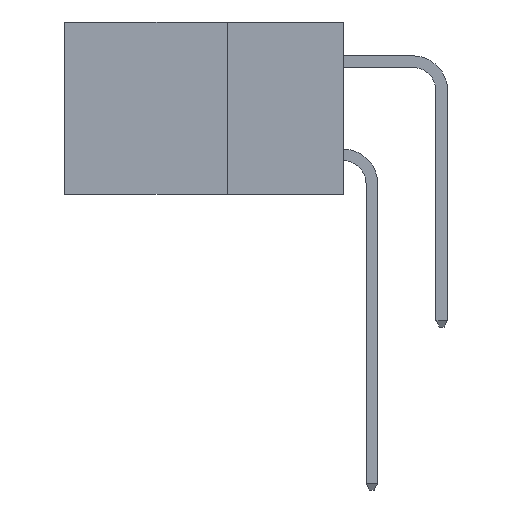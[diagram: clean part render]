
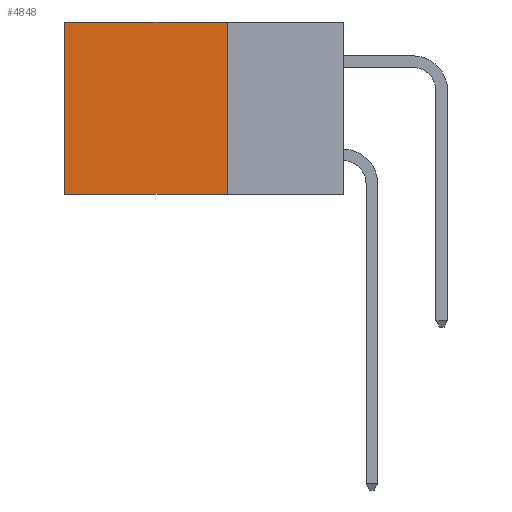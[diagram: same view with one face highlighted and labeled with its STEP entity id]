
A CAD part, left-side view. The second image highlights one B-rep face of the part: STEP entity #4848.
In plain terms, the highlighted planar face has unit normal (-1, 0, 0).
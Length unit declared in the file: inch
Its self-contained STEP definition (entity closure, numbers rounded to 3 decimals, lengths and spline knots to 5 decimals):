
#10 = CARTESIAN_POINT ( 'NONE',  ( 0.2615, 0.6, 0. ) ) ;
#132 = ORIENTED_EDGE ( 'NONE', *, *, #13895, .F. ) ;
#454 = CARTESIAN_POINT ( 'NONE',  ( 0.2615, 0.25, 0. ) ) ;
#584 = ORIENTED_EDGE ( 'NONE', *, *, #7224, .T. ) ;
#1139 = DIRECTION ( 'NONE',  ( 0., 1., 0. ) ) ;
#1399 = VERTEX_POINT ( 'NONE', #11366 ) ;
#1721 = LINE ( 'NONE', #16813, #5251 ) ;
#1735 = LINE ( 'NONE', #15710, #2147 ) ;
#2135 = ORIENTED_EDGE ( 'NONE', *, *, #13456, .T. ) ;
#2147 = VECTOR ( 'NONE', #7978, 39.37008 ) ;
#2763 = LINE ( 'NONE', #3439, #6341 ) ;
#3439 = CARTESIAN_POINT ( 'NONE',  ( 0.2615, 0.25, -0.37 ) ) ;
#4671 = VECTOR ( 'NONE', #10097, 39.37008 ) ;
#4848 = ADVANCED_FACE ( 'NONE', ( #13438 ), #8005, .F. ) ;
#5251 = VECTOR ( 'NONE', #1139, 39.37008 ) ;
#5599 = EDGE_LOOP ( 'NONE', ( #2135, #9221, #132, #584 ) ) ;
#6173 = CARTESIAN_POINT ( 'NONE',  ( 0.2615, 0.6, -0.37 ) ) ;
#6341 = VECTOR ( 'NONE', #11359, 39.37008 ) ;
#7224 = EDGE_CURVE ( 'NONE', #13045, #9764, #15558, .T. ) ;
#7541 = DIRECTION ( 'NONE',  ( 0., 0., -1. ) ) ;
#7622 = DIRECTION ( 'NONE',  ( 1., 0., 0. ) ) ;
#7978 = DIRECTION ( 'NONE',  ( 0., 0., -1. ) ) ;
#8005 = PLANE ( 'NONE',  #13146 ) ;
#8164 = CARTESIAN_POINT ( 'NONE',  ( 0.2615, 0.25, -0.37 ) ) ;
#9221 = ORIENTED_EDGE ( 'NONE', *, *, #14590, .F. ) ;
#9764 = VERTEX_POINT ( 'NONE', #10 ) ;
#9894 = CARTESIAN_POINT ( 'NONE',  ( 0.2615, 0.25, 0. ) ) ;
#10097 = DIRECTION ( 'NONE',  ( 0., 1., 0. ) ) ;
#11359 = DIRECTION ( 'NONE',  ( 0., 0., -1. ) ) ;
#11366 = CARTESIAN_POINT ( 'NONE',  ( 0.2615, 0.25, -0.37 ) ) ;
#13045 = VERTEX_POINT ( 'NONE', #454 ) ;
#13146 = AXIS2_PLACEMENT_3D ( 'NONE', #8164, #7622, #7541 ) ;
#13213 = VERTEX_POINT ( 'NONE', #6173 ) ;
#13438 = FACE_OUTER_BOUND ( 'NONE', #5599, .T. ) ;
#13456 = EDGE_CURVE ( 'NONE', #9764, #13213, #1735, .T. ) ;
#13895 = EDGE_CURVE ( 'NONE', #13045, #1399, #2763, .T. ) ;
#14590 = EDGE_CURVE ( 'NONE', #1399, #13213, #1721, .T. ) ;
#15558 = LINE ( 'NONE', #9894, #4671 ) ;
#15710 = CARTESIAN_POINT ( 'NONE',  ( 0.2615, 0.6, -0.37 ) ) ;
#16813 = CARTESIAN_POINT ( 'NONE',  ( 0.2615, 0.25, -0.37 ) ) ;
